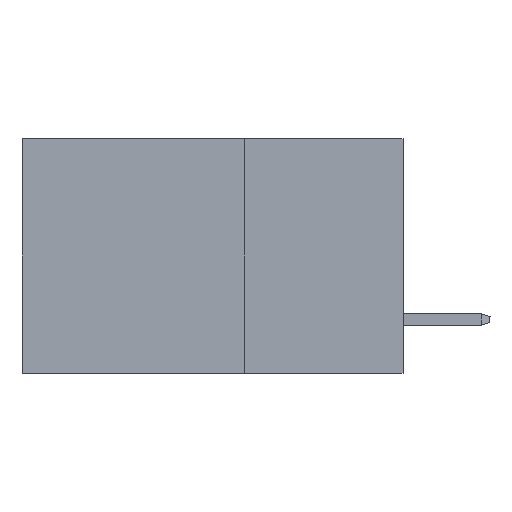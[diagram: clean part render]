
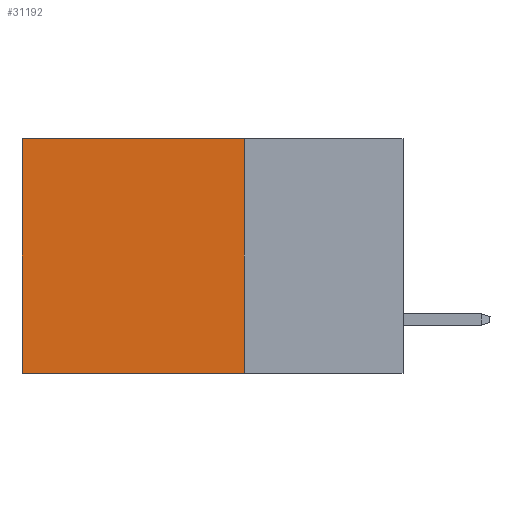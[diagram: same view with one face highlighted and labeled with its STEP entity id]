
A CAD part, left-side view. The second image highlights one B-rep face of the part: STEP entity #31192.
In plain terms, the highlighted planar face has unit normal (-1, 0, 0).
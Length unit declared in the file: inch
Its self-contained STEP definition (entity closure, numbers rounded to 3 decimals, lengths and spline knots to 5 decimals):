
#424 = CARTESIAN_POINT ( 'NONE',  ( 0.2875, 0.6, -0.37 ) ) ;
#1329 = EDGE_CURVE ( 'NONE', #10164, #5439, #25894, .T. ) ;
#2012 = CARTESIAN_POINT ( 'NONE',  ( 0.2875, 0.25, 0. ) ) ;
#2588 = EDGE_CURVE ( 'NONE', #5439, #31711, #27304, .T. ) ;
#3134 = ORIENTED_EDGE ( 'NONE', *, *, #6184, .T. ) ;
#5054 = DIRECTION ( 'NONE',  ( 1., 0., 0. ) ) ;
#5439 = VERTEX_POINT ( 'NONE', #20662 ) ;
#5676 = DIRECTION ( 'NONE',  ( 0., 1., 0. ) ) ;
#6184 = EDGE_CURVE ( 'NONE', #24343, #31711, #30809, .T. ) ;
#6516 = DIRECTION ( 'NONE',  ( 0., 0., -1. ) ) ;
#7691 = CARTESIAN_POINT ( 'NONE',  ( 0.2875, 0.25, 0. ) ) ;
#8818 = CARTESIAN_POINT ( 'NONE',  ( 0.2875, 0.25, 0. ) ) ;
#9344 = DIRECTION ( 'NONE',  ( 0., 1., 0. ) ) ;
#10072 = VECTOR ( 'NONE', #5676, 39.37008 ) ;
#10164 = VERTEX_POINT ( 'NONE', #2012 ) ;
#10693 = AXIS2_PLACEMENT_3D ( 'NONE', #7691, #5054, #21433 ) ;
#12698 = VECTOR ( 'NONE', #6516, 39.37008 ) ;
#12831 = PLANE ( 'NONE',  #10693 ) ;
#14288 = CARTESIAN_POINT ( 'NONE',  ( 0.2875, 0.6, 0. ) ) ;
#16913 = LINE ( 'NONE', #8818, #21486 ) ;
#18706 = CARTESIAN_POINT ( 'NONE',  ( 0.2875, 0.25, -0.37 ) ) ;
#18939 = ORIENTED_EDGE ( 'NONE', *, *, #33940, .T. ) ;
#20043 = ORIENTED_EDGE ( 'NONE', *, *, #1329, .F. ) ;
#20662 = CARTESIAN_POINT ( 'NONE',  ( 0.2875, 0.25, -0.37 ) ) ;
#21064 = FACE_OUTER_BOUND ( 'NONE', #26826, .T. ) ;
#21433 = DIRECTION ( 'NONE',  ( 0., 0., -1. ) ) ;
#21486 = VECTOR ( 'NONE', #9344, 39.37008 ) ;
#22950 = VECTOR ( 'NONE', #31340, 39.37008 ) ;
#23277 = CARTESIAN_POINT ( 'NONE',  ( 0.2875, 0.25, 0. ) ) ;
#24343 = VERTEX_POINT ( 'NONE', #25468 ) ;
#25400 = ORIENTED_EDGE ( 'NONE', *, *, #2588, .F. ) ;
#25468 = CARTESIAN_POINT ( 'NONE',  ( 0.2875, 0.6, 0. ) ) ;
#25894 = LINE ( 'NONE', #23277, #22950 ) ;
#26826 = EDGE_LOOP ( 'NONE', ( #3134, #25400, #20043, #18939 ) ) ;
#27304 = LINE ( 'NONE', #18706, #10072 ) ;
#30809 = LINE ( 'NONE', #14288, #12698 ) ;
#31192 = ADVANCED_FACE ( 'NONE', ( #21064 ), #12831, .F. ) ;
#31340 = DIRECTION ( 'NONE',  ( 0., 0., -1. ) ) ;
#31711 = VERTEX_POINT ( 'NONE', #424 ) ;
#33940 = EDGE_CURVE ( 'NONE', #10164, #24343, #16913, .T. ) ;
